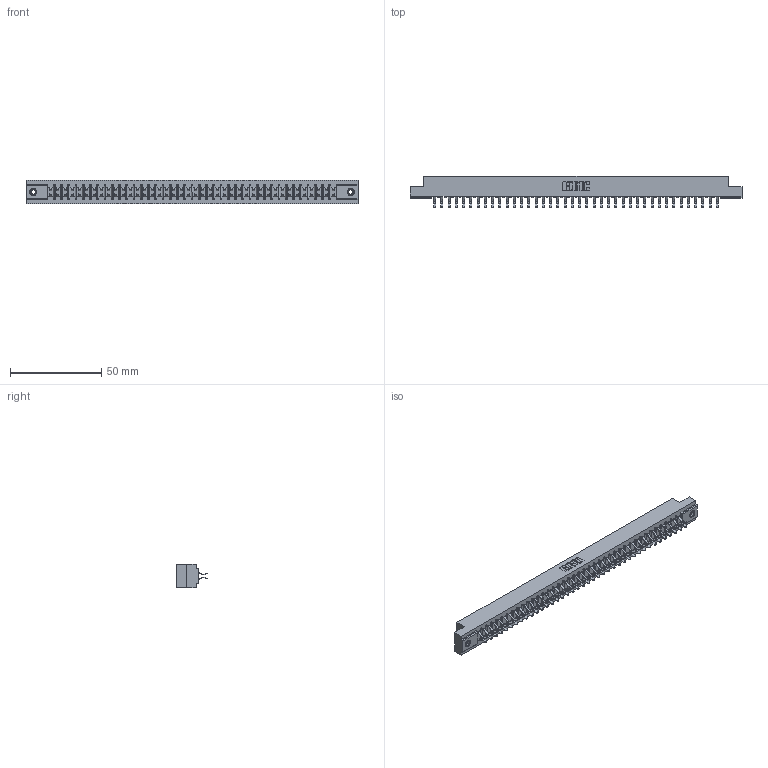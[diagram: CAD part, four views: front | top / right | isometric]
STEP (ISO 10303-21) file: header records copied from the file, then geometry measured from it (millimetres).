
FILE_DESCRIPTION (( 'STEP AP203' ), '1' );
FILE_NAME ('807-080-556-207.STEP', '2021-07-20T16:54:52', ( '' ), ( '' ), 'SwSTEP 2.0', 'SolidWorks 2020', '' );
FILE_SCHEMA (( 'CONFIG_CONTROL_DESIGN' ));
Length unit declared in the file: inch
Products named in the file (4): 307-290-001_556; 807-080-556-207; 345-250-001_345-250-005-103; 807 Part_.156 Dia Mounting Holes
Assembly tree (83 placements, depth 2):
  807-080-556-207
    807 Part_.156 Dia Mounting Holes
    307-290-001_556  x80
    345-250-001_345-250-005-103  x2
Bounding box: 181.51 x 16.97 x 12.7 mm (x, y, z)
Volume: 19259.1 mm3; surface area: 23346.8 mm2
Topology: 83 solids, 83 shells, 4219 faces, 11819 edges, 7654 vertices
Faces by surface type: plane 2742, cylinder 1379, sphere 82, cone 12, torus 4
Entity records: 37107 total; most frequent: CARTESIAN_POINT 6055, ORIENTED_EDGE 5994, DIRECTION 5941, EDGE_CURVE 2997, VECTOR 2297, LINE 2297, VERTEX_POINT 1936, AXIS2_PLACEMENT_3D 1822
